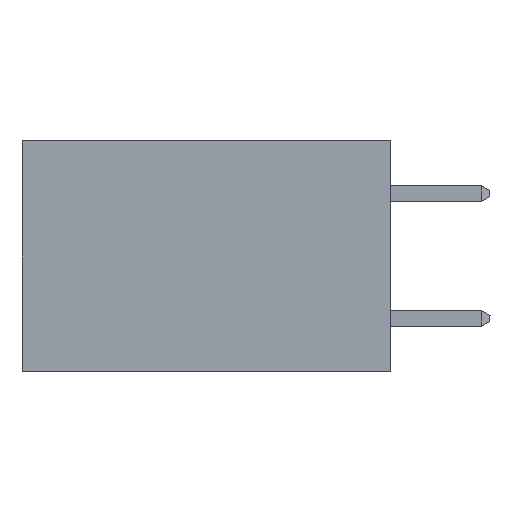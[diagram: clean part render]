
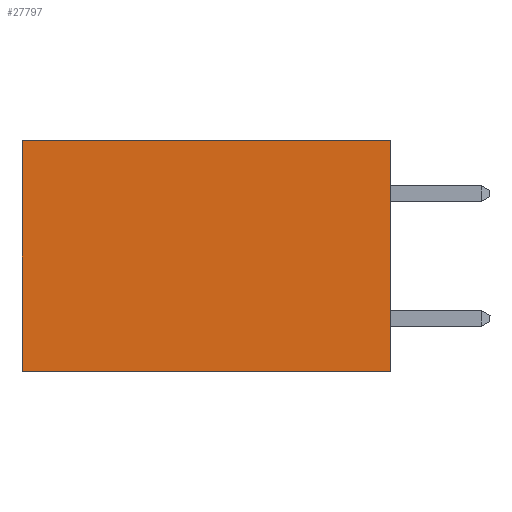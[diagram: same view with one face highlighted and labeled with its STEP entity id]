
A CAD part, left-side view. The second image highlights one B-rep face of the part: STEP entity #27797.
In plain terms, the highlighted planar face has unit normal (-1, 0, 0).
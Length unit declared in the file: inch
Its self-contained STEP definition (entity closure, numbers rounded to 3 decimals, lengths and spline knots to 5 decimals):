
#351 = CARTESIAN_POINT ( 'NONE',  ( 0.277, 0.59, -0.37 ) ) ;
#893 = VECTOR ( 'NONE', #11463, 39.37008 ) ;
#1073 = ORIENTED_EDGE ( 'NONE', *, *, #27502, .T. ) ;
#1279 = CARTESIAN_POINT ( 'NONE',  ( 0.277, 0., -0.37 ) ) ;
#2888 = ORIENTED_EDGE ( 'NONE', *, *, #8944, .F. ) ;
#3616 = VERTEX_POINT ( 'NONE', #5770 ) ;
#5770 = CARTESIAN_POINT ( 'NONE',  ( 0.277, 0., 0. ) ) ;
#7038 = CARTESIAN_POINT ( 'NONE',  ( 0.277, 0.59, 0. ) ) ;
#7510 = LINE ( 'NONE', #31510, #26935 ) ;
#7981 = FACE_OUTER_BOUND ( 'NONE', #21819, .T. ) ;
#8944 = EDGE_CURVE ( 'NONE', #21303, #12380, #32293, .T. ) ;
#8979 = CARTESIAN_POINT ( 'NONE',  ( 0.277, 0., -0.37 ) ) ;
#9295 = ORIENTED_EDGE ( 'NONE', *, *, #12813, .F. ) ;
#10431 = CARTESIAN_POINT ( 'NONE',  ( 0.277, 0.59, -0.37 ) ) ;
#11463 = DIRECTION ( 'NONE',  ( 0., 0., -1. ) ) ;
#11514 = DIRECTION ( 'NONE',  ( 0., 0., -1. ) ) ;
#12043 = VECTOR ( 'NONE', #27279, 39.37008 ) ;
#12380 = VERTEX_POINT ( 'NONE', #10431 ) ;
#12813 = EDGE_CURVE ( 'NONE', #3616, #21303, #21128, .T. ) ;
#13731 = DIRECTION ( 'NONE',  ( 0., 1., 0. ) ) ;
#16707 = ORIENTED_EDGE ( 'NONE', *, *, #29949, .T. ) ;
#17905 = VERTEX_POINT ( 'NONE', #7038 ) ;
#20643 = DIRECTION ( 'NONE',  ( 0., 0., -1. ) ) ;
#21128 = LINE ( 'NONE', #1279, #893 ) ;
#21303 = VERTEX_POINT ( 'NONE', #29240 ) ;
#21625 = PLANE ( 'NONE',  #25496 ) ;
#21819 = EDGE_LOOP ( 'NONE', ( #1073, #2888, #9295, #16707 ) ) ;
#23484 = VECTOR ( 'NONE', #20643, 39.37008 ) ;
#25496 = AXIS2_PLACEMENT_3D ( 'NONE', #8979, #26708, #11514 ) ;
#26708 = DIRECTION ( 'NONE',  ( 1., 0., 0. ) ) ;
#26935 = VECTOR ( 'NONE', #13731, 39.37008 ) ;
#27279 = DIRECTION ( 'NONE',  ( 0., 1., 0. ) ) ;
#27502 = EDGE_CURVE ( 'NONE', #17905, #12380, #30236, .T. ) ;
#27797 = ADVANCED_FACE ( 'NONE', ( #7981 ), #21625, .F. ) ;
#29240 = CARTESIAN_POINT ( 'NONE',  ( 0.277, 0., -0.37 ) ) ;
#29428 = CARTESIAN_POINT ( 'NONE',  ( 0.277, 0., -0.37 ) ) ;
#29949 = EDGE_CURVE ( 'NONE', #3616, #17905, #7510, .T. ) ;
#30236 = LINE ( 'NONE', #351, #23484 ) ;
#31510 = CARTESIAN_POINT ( 'NONE',  ( 0.277, 0., 0. ) ) ;
#32293 = LINE ( 'NONE', #29428, #12043 ) ;
